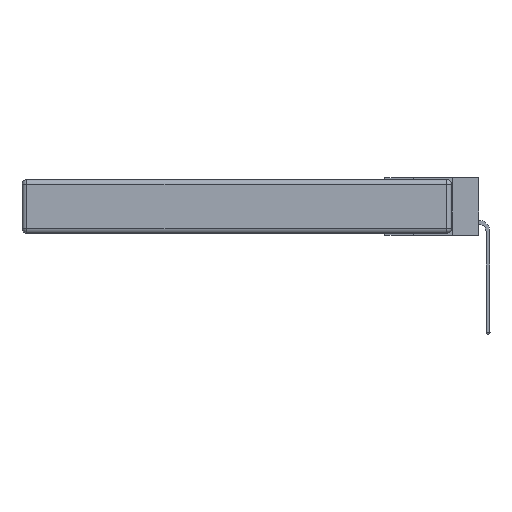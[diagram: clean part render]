
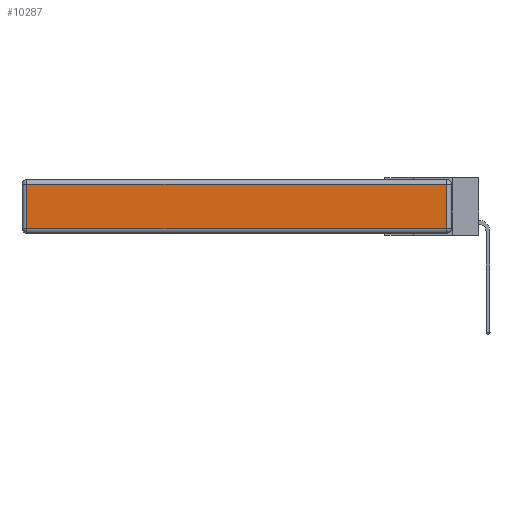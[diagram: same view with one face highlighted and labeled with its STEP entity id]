
A CAD part, left-side view. The second image highlights one B-rep face of the part: STEP entity #10287.
In plain terms, the highlighted planar face has unit normal (-1, 0, 0).
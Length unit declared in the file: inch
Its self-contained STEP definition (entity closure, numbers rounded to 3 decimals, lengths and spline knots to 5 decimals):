
#611 = CARTESIAN_POINT ( 'NONE',  ( 0., 2.72, -0.03 ) ) ;
#722 = DIRECTION ( 'NONE',  ( 0., 0., 1. ) ) ;
#768 = CARTESIAN_POINT ( 'NONE',  ( 0., 0.03, -0.313 ) ) ;
#769 = PLANE ( 'NONE',  #4825 ) ;
#842 = EDGE_CURVE ( 'NONE', #9456, #5947, #1851, .T. ) ;
#1707 = VECTOR ( 'NONE', #2829, 39.37008 ) ;
#1851 = LINE ( 'NONE', #12301, #5553 ) ;
#1956 = FACE_OUTER_BOUND ( 'NONE', #8351, .T. ) ;
#2058 = VERTEX_POINT ( 'NONE', #11991 ) ;
#2659 = CARTESIAN_POINT ( 'NONE',  ( 0., 0., -0.343 ) ) ;
#2829 = DIRECTION ( 'NONE',  ( 0., 0., -1. ) ) ;
#3004 = ORIENTED_EDGE ( 'NONE', *, *, #842, .T. ) ;
#3488 = EDGE_CURVE ( 'NONE', #2058, #7771, #6069, .T. ) ;
#4532 = CARTESIAN_POINT ( 'NONE',  ( 0., 0.03, -0.343 ) ) ;
#4584 = EDGE_CURVE ( 'NONE', #7771, #9456, #12652, .T. ) ;
#4825 = AXIS2_PLACEMENT_3D ( 'NONE', #2659, #9811, #722 ) ;
#5361 = CARTESIAN_POINT ( 'NONE',  ( 0., 2.72, -0.313 ) ) ;
#5553 = VECTOR ( 'NONE', #13236, 39.37008 ) ;
#5632 = LINE ( 'NONE', #4532, #8665 ) ;
#5947 = VERTEX_POINT ( 'NONE', #768 ) ;
#6069 = LINE ( 'NONE', #11474, #12358 ) ;
#6716 = CARTESIAN_POINT ( 'NONE',  ( 0., 2.72, -0.343 ) ) ;
#7771 = VERTEX_POINT ( 'NONE', #611 ) ;
#8329 = ORIENTED_EDGE ( 'NONE', *, *, #3488, .T. ) ;
#8351 = EDGE_LOOP ( 'NONE', ( #3004, #10677, #8329, #10595 ) ) ;
#8665 = VECTOR ( 'NONE', #12621, 39.37008 ) ;
#9456 = VERTEX_POINT ( 'NONE', #5361 ) ;
#9811 = DIRECTION ( 'NONE',  ( -1., 0., 0. ) ) ;
#10287 = ADVANCED_FACE ( 'NONE', ( #1956 ), #769, .T. ) ;
#10595 = ORIENTED_EDGE ( 'NONE', *, *, #4584, .T. ) ;
#10677 = ORIENTED_EDGE ( 'NONE', *, *, #11836, .T. ) ;
#11474 = CARTESIAN_POINT ( 'NONE',  ( 0., 2.75, -0.03 ) ) ;
#11836 = EDGE_CURVE ( 'NONE', #5947, #2058, #5632, .T. ) ;
#11991 = CARTESIAN_POINT ( 'NONE',  ( 0., 0.03, -0.03 ) ) ;
#12301 = CARTESIAN_POINT ( 'NONE',  ( 0., 0., -0.313 ) ) ;
#12358 = VECTOR ( 'NONE', #12457, 39.37008 ) ;
#12457 = DIRECTION ( 'NONE',  ( 0., 1., 0. ) ) ;
#12621 = DIRECTION ( 'NONE',  ( 0., 0., 1. ) ) ;
#12652 = LINE ( 'NONE', #6716, #1707 ) ;
#13236 = DIRECTION ( 'NONE',  ( 0., -1., 0. ) ) ;
